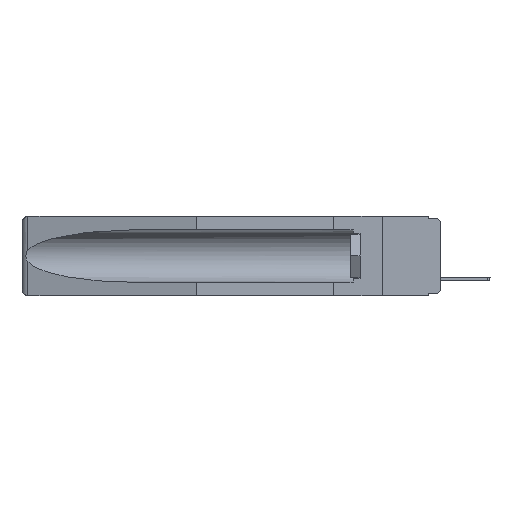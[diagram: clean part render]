
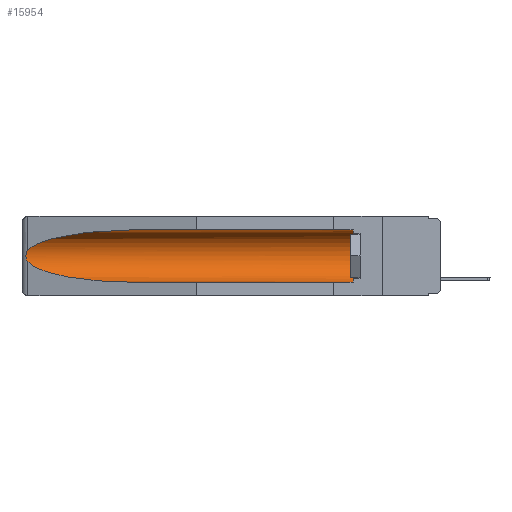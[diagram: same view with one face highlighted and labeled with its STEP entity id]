
A CAD part, left-side view. The second image highlights one B-rep face of the part: STEP entity #15954.
In plain terms, the highlighted cylindrical face has radius 2.857 mm (diameter 5.715 mm), a partial arc.
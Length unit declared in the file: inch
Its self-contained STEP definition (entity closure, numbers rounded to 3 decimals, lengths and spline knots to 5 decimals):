
#293 = ORIENTED_EDGE ( 'NONE', *, *, #9690, .T. ) ;
#380 = CARTESIAN_POINT ( 'NONE',  ( 0.26597, 1.5296, -0.19026 ) ) ;
#446 = CARTESIAN_POINT ( 'NONE',  ( 0.26654, 1.53092, -0.15636 ) ) ;
#685 = CARTESIAN_POINT ( 'NONE',  ( 0.155, 1.07973, -0.284 ) ) ;
#686 = VERTEX_POINT ( 'NONE', #15646 ) ;
#977 = VERTEX_POINT ( 'NONE', #17070 ) ;
#1187 = ORIENTED_EDGE ( 'NONE', *, *, #1950, .T. ) ;
#1280 = LINE ( 'NONE', #16914, #6654 ) ;
#1652 = EDGE_LOOP ( 'NONE', ( #1816, #12889, #16175, #13379, #1187, #293 ) ) ;
#1717 = DIRECTION ( 'NONE',  ( 0., 0., 1. ) ) ;
#1779 = DIRECTION ( 'NONE',  ( 0., 1., 0. ) ) ;
#1786 = CARTESIAN_POINT ( 'NONE',  ( 0.25451, 1.48313, -0.09465 ) ) ;
#1816 = ORIENTED_EDGE ( 'NONE', *, *, #12197, .T. ) ;
#1950 = EDGE_CURVE ( 'NONE', #12853, #9773, #10963, .T. ) ;
#2029 = CARTESIAN_POINT ( 'NONE',  ( 0.155, -0.30754, -0.1715 ) ) ;
#2569 = CARTESIAN_POINT ( 'NONE',  ( 0.155, 0.126, -0.059 ) ) ;
#3068 =( BOUNDED_CURVE ( )  B_SPLINE_CURVE ( 3, ( #3385, #4771, #8938, #685 ),
 .UNSPECIFIED., .F., .T. ) 
 B_SPLINE_CURVE_WITH_KNOTS ( ( 4, 4 ),
 ( 0.1948, 1.5708 ),
 .UNSPECIFIED. ) 
 CURVE ( )  GEOMETRIC_REPRESENTATION_ITEM ( )  RATIONAL_B_SPLINE_CURVE ( ( 1., 0.848, 0.848, 1. ) ) 
 REPRESENTATION_ITEM ( '' )  );
#3151 = CARTESIAN_POINT ( 'NONE',  ( 0.2673, 1.5327, -0.16383 ) ) ;
#3385 = CARTESIAN_POINT ( 'NONE',  ( 0.26537, 1.52718, -0.19328 ) ) ;
#4379 = CARTESIAN_POINT ( 'NONE',  ( 0.21114, 1.30732, -0.059 ) ) ;
#4435 = CARTESIAN_POINT ( 'NONE',  ( 0.155, 1.07973, -0.059 ) ) ;
#4589 = CYLINDRICAL_SURFACE ( 'NONE', #15840, 0.1125 ) ;
#4771 = CARTESIAN_POINT ( 'NONE',  ( 0.25451, 1.48313, -0.24835 ) ) ;
#5779 = EDGE_CURVE ( 'NONE', #14244, #977, #7555, .T. ) ;
#5865 = DIRECTION ( 'NONE',  ( 0., -1., 0. ) ) ;
#6300 = DIRECTION ( 'NONE',  ( 0., 1., 0. ) ) ;
#6654 = VECTOR ( 'NONE', #1779, 39.37008 ) ;
#6960 = FACE_OUTER_BOUND ( 'NONE', #1652, .T. ) ;
#7153 = CARTESIAN_POINT ( 'NONE',  ( 0.2673, 1.53269, -0.17917 ) ) ;
#7555 = B_SPLINE_CURVE_WITH_KNOTS ( 'NONE', 3,
 ( #11373, #14208, #446, #3151, #17021, #8741, #7153, #8567, #380, #16900 ),
 .UNSPECIFIED., .F., .F.,
 ( 4, 2, 2, 2, 4 ),
 ( 0., 0.00029, 0.00058, 0.00087, 0.00117 ),
 .UNSPECIFIED. ) ;
#7595 = EDGE_CURVE ( 'NONE', #12853, #10989, #1280, .T. ) ;
#7865 = CARTESIAN_POINT ( 'NONE',  ( 0.26537, 1.52718, -0.14972 ) ) ;
#8129 =( BOUNDED_CURVE ( )  B_SPLINE_CURVE ( 3, ( #4435, #4379, #1786, #15375 ),
 .UNSPECIFIED., .F., .F. ) 
 B_SPLINE_CURVE_WITH_KNOTS ( ( 4, 4 ),
 ( 4.71239, 6.08839 ),
 .UNSPECIFIED. ) 
 CURVE ( )  GEOMETRIC_REPRESENTATION_ITEM ( )  RATIONAL_B_SPLINE_CURVE ( ( 1., 0.848, 0.848, 1. ) ) 
 REPRESENTATION_ITEM ( '' )  );
#8220 = CARTESIAN_POINT ( 'NONE',  ( 0.155, 0.126, -0.284 ) ) ;
#8496 = LINE ( 'NONE', #11878, #15846 ) ;
#8567 = CARTESIAN_POINT ( 'NONE',  ( 0.26655, 1.53094, -0.18657 ) ) ;
#8741 = CARTESIAN_POINT ( 'NONE',  ( 0.2675, 1.53308, -0.17534 ) ) ;
#8938 = CARTESIAN_POINT ( 'NONE',  ( 0.21114, 1.30732, -0.284 ) ) ;
#9690 = EDGE_CURVE ( 'NONE', #9773, #686, #8496, .T. ) ;
#9773 = VERTEX_POINT ( 'NONE', #2569 ) ;
#10963 = CIRCLE ( 'NONE', #12025, 0.1125 ) ;
#10989 = VERTEX_POINT ( 'NONE', #12307 ) ;
#11369 = EDGE_CURVE ( 'NONE', #977, #10989, #3068, .T. ) ;
#11373 = CARTESIAN_POINT ( 'NONE',  ( 0.26537, 1.52718, -0.14972 ) ) ;
#11511 = CARTESIAN_POINT ( 'NONE',  ( 0.155, 0.126, -0.1715 ) ) ;
#11878 = CARTESIAN_POINT ( 'NONE',  ( 0.155, -0.30754, -0.059 ) ) ;
#12005 = DIRECTION ( 'NONE',  ( 0., 1., 0. ) ) ;
#12025 = AXIS2_PLACEMENT_3D ( 'NONE', #11511, #5865, #1717 ) ;
#12197 = EDGE_CURVE ( 'NONE', #686, #14244, #8129, .T. ) ;
#12307 = CARTESIAN_POINT ( 'NONE',  ( 0.155, 1.07973, -0.284 ) ) ;
#12853 = VERTEX_POINT ( 'NONE', #8220 ) ;
#12889 = ORIENTED_EDGE ( 'NONE', *, *, #5779, .T. ) ;
#13283 = DIRECTION ( 'NONE',  ( 0., 0., 1. ) ) ;
#13379 = ORIENTED_EDGE ( 'NONE', *, *, #7595, .F. ) ;
#14208 = CARTESIAN_POINT ( 'NONE',  ( 0.26597, 1.52961, -0.15275 ) ) ;
#14244 = VERTEX_POINT ( 'NONE', #7865 ) ;
#15375 = CARTESIAN_POINT ( 'NONE',  ( 0.26537, 1.52718, -0.14972 ) ) ;
#15646 = CARTESIAN_POINT ( 'NONE',  ( 0.155, 1.07973, -0.059 ) ) ;
#15840 = AXIS2_PLACEMENT_3D ( 'NONE', #2029, #6300, #13283 ) ;
#15846 = VECTOR ( 'NONE', #12005, 39.37008 ) ;
#15954 = ADVANCED_FACE ( 'NONE', ( #6960 ), #4589, .F. ) ;
#16175 = ORIENTED_EDGE ( 'NONE', *, *, #11369, .T. ) ;
#16900 = CARTESIAN_POINT ( 'NONE',  ( 0.26537, 1.52718, -0.19328 ) ) ;
#16914 = CARTESIAN_POINT ( 'NONE',  ( 0.155, -0.30754, -0.284 ) ) ;
#17021 = CARTESIAN_POINT ( 'NONE',  ( 0.2675, 1.53308, -0.16763 ) ) ;
#17070 = CARTESIAN_POINT ( 'NONE',  ( 0.26537, 1.52718, -0.19328 ) ) ;
